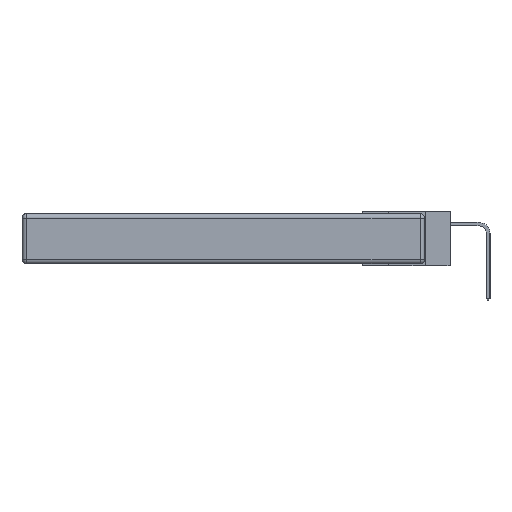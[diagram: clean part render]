
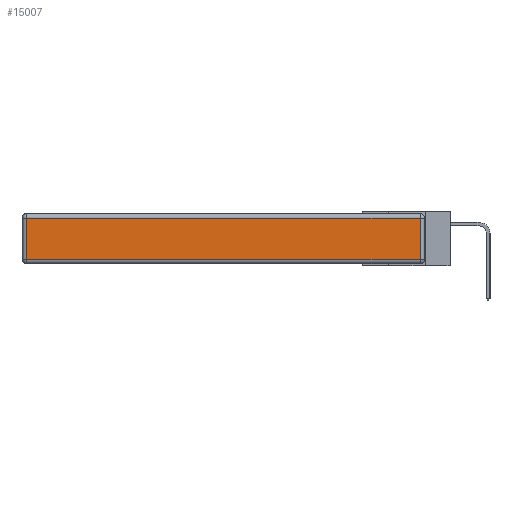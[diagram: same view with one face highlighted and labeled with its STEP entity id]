
A CAD part, left-side view. The second image highlights one B-rep face of the part: STEP entity #15007.
In plain terms, the highlighted planar face has unit normal (-1, 0, 0).
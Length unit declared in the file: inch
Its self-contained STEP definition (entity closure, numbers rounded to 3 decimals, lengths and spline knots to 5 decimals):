
#140 = LINE ( 'NONE', #7797, #1513 ) ;
#1300 = CARTESIAN_POINT ( 'NONE',  ( 0., 0., -0.313 ) ) ;
#1422 = AXIS2_PLACEMENT_3D ( 'NONE', #9267, #10798, #7096 ) ;
#1513 = VECTOR ( 'NONE', #1888, 39.37008 ) ;
#1529 = CARTESIAN_POINT ( 'NONE',  ( 0., 0.03, -0.03 ) ) ;
#1888 = DIRECTION ( 'NONE',  ( 0., 1., 0. ) ) ;
#4399 = VERTEX_POINT ( 'NONE', #12206 ) ;
#4737 = ORIENTED_EDGE ( 'NONE', *, *, #7266, .T. ) ;
#5518 = EDGE_CURVE ( 'NONE', #4399, #5811, #12068, .T. ) ;
#5811 = VERTEX_POINT ( 'NONE', #1529 ) ;
#6347 = EDGE_CURVE ( 'NONE', #5811, #15182, #140, .T. ) ;
#7026 = LINE ( 'NONE', #8368, #15769 ) ;
#7096 = DIRECTION ( 'NONE',  ( 0., 0., 1. ) ) ;
#7266 = EDGE_CURVE ( 'NONE', #15182, #9936, #7026, .T. ) ;
#7387 = ORIENTED_EDGE ( 'NONE', *, *, #5518, .T. ) ;
#7797 = CARTESIAN_POINT ( 'NONE',  ( 0., 2.75, -0.03 ) ) ;
#8245 = DIRECTION ( 'NONE',  ( 0., 0., 1. ) ) ;
#8368 = CARTESIAN_POINT ( 'NONE',  ( 0., 2.72, -0.343 ) ) ;
#8681 = VECTOR ( 'NONE', #8245, 39.37008 ) ;
#8815 = EDGE_CURVE ( 'NONE', #9936, #4399, #9332, .T. ) ;
#9009 = DIRECTION ( 'NONE',  ( 0., -1., 0. ) ) ;
#9267 = CARTESIAN_POINT ( 'NONE',  ( 0., 0., -0.343 ) ) ;
#9332 = LINE ( 'NONE', #1300, #15858 ) ;
#9650 = DIRECTION ( 'NONE',  ( 0., 0., -1. ) ) ;
#9936 = VERTEX_POINT ( 'NONE', #12512 ) ;
#10798 = DIRECTION ( 'NONE',  ( -1., 0., 0. ) ) ;
#12068 = LINE ( 'NONE', #14537, #8681 ) ;
#12206 = CARTESIAN_POINT ( 'NONE',  ( 0., 0.03, -0.313 ) ) ;
#12512 = CARTESIAN_POINT ( 'NONE',  ( 0., 2.72, -0.313 ) ) ;
#12588 = FACE_OUTER_BOUND ( 'NONE', #14037, .T. ) ;
#12932 = ORIENTED_EDGE ( 'NONE', *, *, #8815, .T. ) ;
#14037 = EDGE_LOOP ( 'NONE', ( #12932, #7387, #15336, #4737 ) ) ;
#14287 = PLANE ( 'NONE',  #1422 ) ;
#14537 = CARTESIAN_POINT ( 'NONE',  ( 0., 0.03, -0.343 ) ) ;
#14887 = CARTESIAN_POINT ( 'NONE',  ( 0., 2.72, -0.03 ) ) ;
#15007 = ADVANCED_FACE ( 'NONE', ( #12588 ), #14287, .T. ) ;
#15182 = VERTEX_POINT ( 'NONE', #14887 ) ;
#15336 = ORIENTED_EDGE ( 'NONE', *, *, #6347, .T. ) ;
#15769 = VECTOR ( 'NONE', #9650, 39.37008 ) ;
#15858 = VECTOR ( 'NONE', #9009, 39.37008 ) ;
